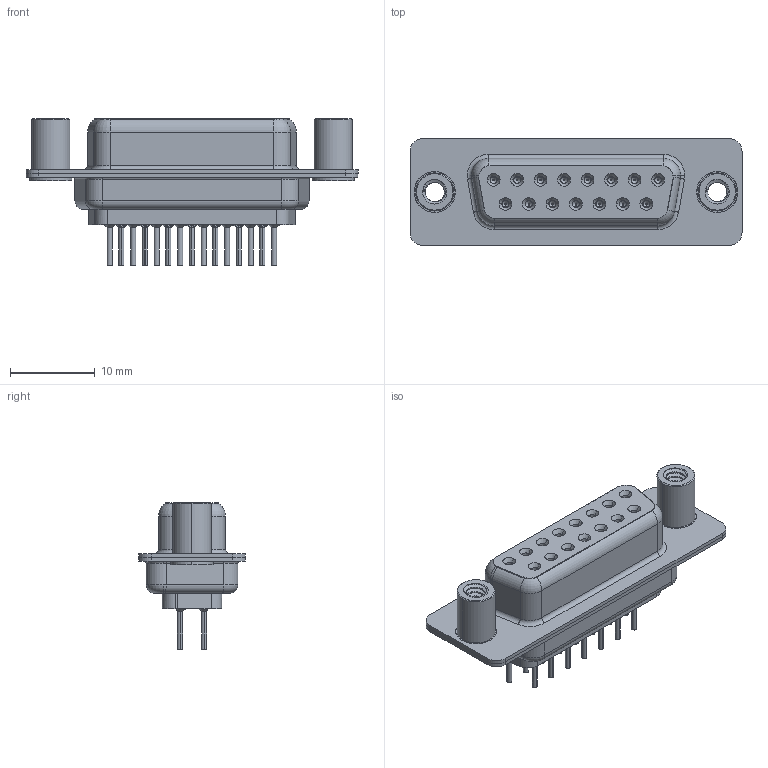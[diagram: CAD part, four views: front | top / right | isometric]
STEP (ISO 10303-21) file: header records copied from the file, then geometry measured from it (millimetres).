
FILE_DESCRIPTION (( 'STEP AP203' ), '1' );
FILE_NAME ('628-015-320-248.STEP', '2020-07-14T01:12:56', ( '' ), ( '' ), 'SwSTEP 2.0', 'SolidWorks 2020', '' );
FILE_SCHEMA (( 'CONFIG_CONTROL_DESIGN' ));
Length unit declared in the file: millimetre
Products named in the file (7): 628-015-320-248; 628 Contact Row 1_20L; 628 Shell Rear_15 Contacts; 628 4-40 Threaded Standoff; 628 Contact Row 2_20L; 628 Shell Front_15 Contacts; 628 Housing_15 LP
Assembly tree (20 placements, depth 2):
  628-015-320-248
    628 Housing_15 LP
    628 Shell Front_15 Contacts
    628 Shell Rear_15 Contacts
    628 Contact Row 1_20L  x8
    628 Contact Row 2_20L  x7
    628 4-40 Threaded Standoff  x2
Bounding box: 39.15 x 12.6 x 17.3 mm (x, y, z)
Volume: 2607 mm3; surface area: 6525.3 mm2
Topology: 20 solids, 20 shells, 2218 faces, 5639 edges, 3504 vertices
Faces by surface type: cylinder 660, plane 534, torus 453, bspline 306, cone 265
Entity records: 24800 total; most frequent: CARTESIAN_POINT 7738, DIRECTION 3445, ORIENTED_EDGE 3306, EDGE_CURVE 1653, AXIS2_PLACEMENT_3D 1431, VERTEX_POINT 1038, EDGE_LOOP 781, CIRCLE 769
